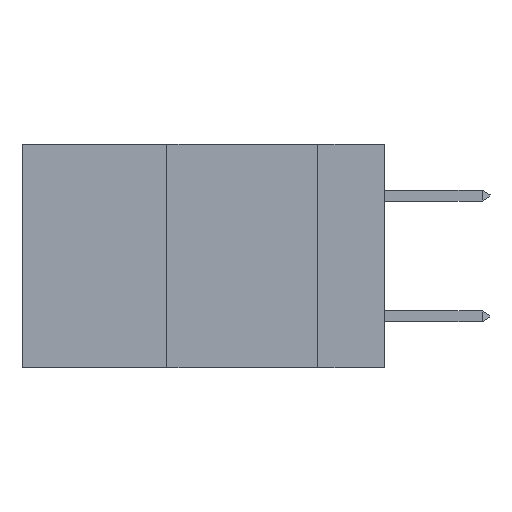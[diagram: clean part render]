
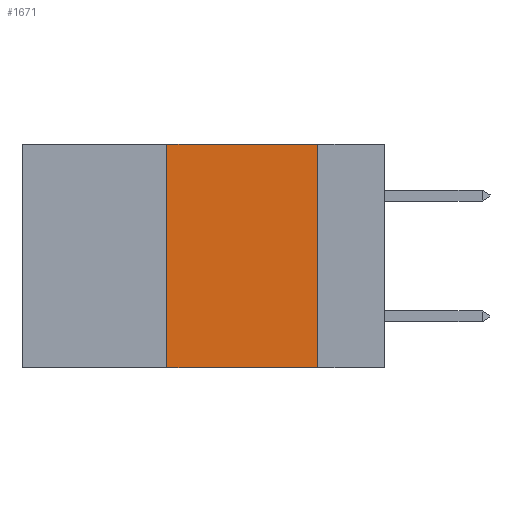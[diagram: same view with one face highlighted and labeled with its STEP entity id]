
A CAD part, left-side view. The second image highlights one B-rep face of the part: STEP entity #1671.
In plain terms, the highlighted planar face has unit normal (-1, 0, 0).
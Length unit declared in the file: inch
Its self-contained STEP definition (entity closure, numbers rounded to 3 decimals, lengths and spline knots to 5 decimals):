
#743 = CARTESIAN_POINT ( 'NONE',  ( 0., 0.6, -0.37 ) ) ;
#1671 = ADVANCED_FACE ( 'NONE', ( #8071 ), #4262, .F. ) ;
#2965 = CARTESIAN_POINT ( 'NONE',  ( 0., 0.36, -0.37 ) ) ;
#3154 = ORIENTED_EDGE ( 'NONE', *, *, #8290, .F. ) ;
#3494 = EDGE_LOOP ( 'NONE', ( #3154, #10537, #8955, #15356 ) ) ;
#4262 = PLANE ( 'NONE',  #8795 ) ;
#4446 = DIRECTION ( 'NONE',  ( 1., 0., 0. ) ) ;
#5227 = VERTEX_POINT ( 'NONE', #2965 ) ;
#5850 = LINE ( 'NONE', #5926, #6331 ) ;
#5926 = CARTESIAN_POINT ( 'NONE',  ( 0., 0.36, 0. ) ) ;
#6331 = VECTOR ( 'NONE', #14740, 39.37008 ) ;
#6662 = VERTEX_POINT ( 'NONE', #11083 ) ;
#6990 = DIRECTION ( 'NONE',  ( 0., -1., 0. ) ) ;
#7626 = VECTOR ( 'NONE', #15268, 39.37008 ) ;
#8071 = FACE_OUTER_BOUND ( 'NONE', #3494, .T. ) ;
#8290 = EDGE_CURVE ( 'NONE', #6662, #10764, #16366, .T. ) ;
#8635 = DIRECTION ( 'NONE',  ( 0., -1., 0. ) ) ;
#8795 = AXIS2_PLACEMENT_3D ( 'NONE', #13241, #4446, #14441 ) ;
#8911 = VECTOR ( 'NONE', #6990, 39.37008 ) ;
#8955 = ORIENTED_EDGE ( 'NONE', *, *, #9709, .F. ) ;
#9220 = CARTESIAN_POINT ( 'NONE',  ( 0., 0.11, -0.37 ) ) ;
#9328 = CARTESIAN_POINT ( 'NONE',  ( 0., 0.36, 0. ) ) ;
#9709 = EDGE_CURVE ( 'NONE', #5227, #16651, #5850, .T. ) ;
#9834 = LINE ( 'NONE', #743, #14640 ) ;
#10537 = ORIENTED_EDGE ( 'NONE', *, *, #12643, .F. ) ;
#10764 = VERTEX_POINT ( 'NONE', #9220 ) ;
#11083 = CARTESIAN_POINT ( 'NONE',  ( 0., 0.11, 0. ) ) ;
#11228 = CARTESIAN_POINT ( 'NONE',  ( 0., 0.6, 0. ) ) ;
#12643 = EDGE_CURVE ( 'NONE', #16651, #6662, #13515, .T. ) ;
#13241 = CARTESIAN_POINT ( 'NONE',  ( 0., 0.6, 0. ) ) ;
#13515 = LINE ( 'NONE', #11228, #8911 ) ;
#14294 = CARTESIAN_POINT ( 'NONE',  ( 0., 0.11, 0. ) ) ;
#14441 = DIRECTION ( 'NONE',  ( 0., 0., -1. ) ) ;
#14640 = VECTOR ( 'NONE', #8635, 39.37008 ) ;
#14695 = EDGE_CURVE ( 'NONE', #5227, #10764, #9834, .T. ) ;
#14740 = DIRECTION ( 'NONE',  ( 0., 0., 1. ) ) ;
#15268 = DIRECTION ( 'NONE',  ( 0., 0., -1. ) ) ;
#15356 = ORIENTED_EDGE ( 'NONE', *, *, #14695, .T. ) ;
#16366 = LINE ( 'NONE', #14294, #7626 ) ;
#16651 = VERTEX_POINT ( 'NONE', #9328 ) ;
